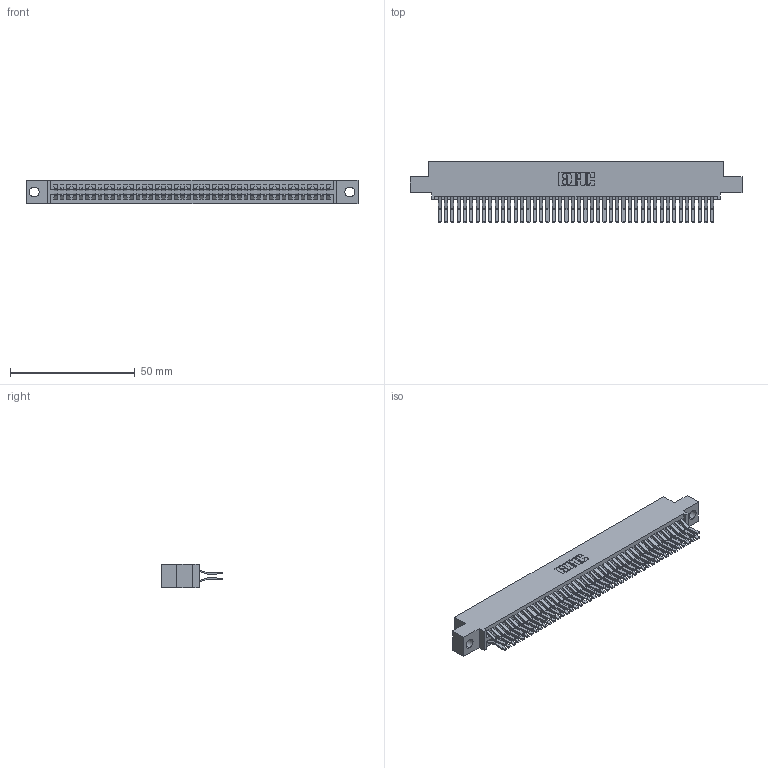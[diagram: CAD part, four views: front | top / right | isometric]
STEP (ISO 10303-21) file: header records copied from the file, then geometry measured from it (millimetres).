
FILE_DESCRIPTION (( 'STEP AP203' ), '1' );
FILE_NAME ('395-088-560-504.STEP', '2018-11-29T02:02:38', ( '' ), ( '' ), 'SwSTEP 2.0', 'SolidWorks 2016', '' );
FILE_SCHEMA (( 'CONFIG_CONTROL_DESIGN' ));
Length unit declared in the file: inch
Products named in the file (3): 345 Part_0.110 Offset - 0.156 Dia-TH; 395-088-560-504; 345-292-001_560 Tail
Assembly tree (89 placements, depth 2):
  395-088-560-504
    345 Part_0.110 Offset - 0.156 Dia-TH
    345-292-001_560 Tail  x88
Bounding box: 132.97 x 24.45 x 9.4 mm (x, y, z)
Volume: 13350.9 mm3; surface area: 21165.1 mm2
Topology: 89 solids, 89 shells, 4706 faces, 13993 edges, 9210 vertices
Faces by surface type: plane 2988, cylinder 1718
Entity records: 34477 total; most frequent: CARTESIAN_POINT 5780, ORIENTED_EDGE 5714, DIRECTION 5097, EDGE_CURVE 2857, LINE 2545, VECTOR 2545, VERTEX_POINT 1902, AXIS2_PLACEMENT_3D 1276
